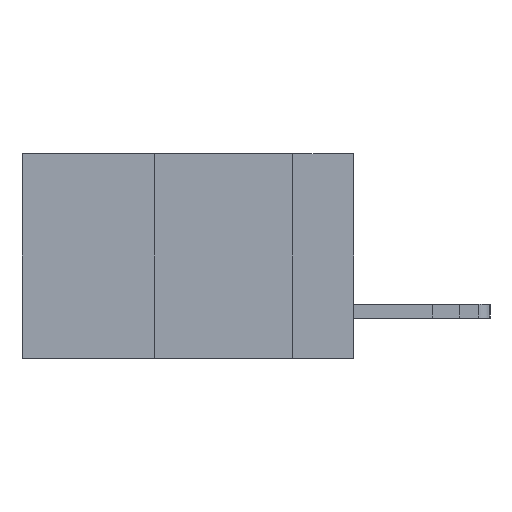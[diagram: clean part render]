
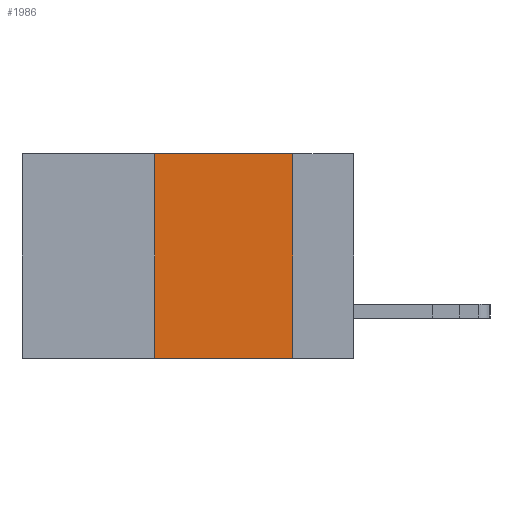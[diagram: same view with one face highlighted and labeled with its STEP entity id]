
A CAD part, left-side view. The second image highlights one B-rep face of the part: STEP entity #1986.
In plain terms, the highlighted planar face has unit normal (-1, 0, 0).
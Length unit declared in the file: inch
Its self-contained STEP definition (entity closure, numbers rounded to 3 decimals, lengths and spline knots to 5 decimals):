
#179 = LINE ( 'NONE', #14898, #10579 ) ;
#461 = ORIENTED_EDGE ( 'NONE', *, *, #7625, .F. ) ;
#1543 = FACE_OUTER_BOUND ( 'NONE', #2567, .T. ) ;
#1986 = ADVANCED_FACE ( 'NONE', ( #1543 ), #6241, .F. ) ;
#2121 = CARTESIAN_POINT ( 'NONE',  ( 0., 0.36, 0. ) ) ;
#2534 = EDGE_CURVE ( 'NONE', #13975, #15255, #6338, .T. ) ;
#2567 = EDGE_LOOP ( 'NONE', ( #5828, #4543, #461, #7724 ) ) ;
#2624 = DIRECTION ( 'NONE',  ( 1., 0., 0. ) ) ;
#3482 = VERTEX_POINT ( 'NONE', #6280 ) ;
#4543 = ORIENTED_EDGE ( 'NONE', *, *, #2534, .F. ) ;
#5828 = ORIENTED_EDGE ( 'NONE', *, *, #9604, .F. ) ;
#6241 = PLANE ( 'NONE',  #15518 ) ;
#6280 = CARTESIAN_POINT ( 'NONE',  ( 0., 0.11, -0.37 ) ) ;
#6338 = LINE ( 'NONE', #11328, #13417 ) ;
#6560 = CARTESIAN_POINT ( 'NONE',  ( 0., 0.6, 0. ) ) ;
#7625 = EDGE_CURVE ( 'NONE', #9426, #13975, #9489, .T. ) ;
#7724 = ORIENTED_EDGE ( 'NONE', *, *, #10273, .T. ) ;
#7765 = VECTOR ( 'NONE', #13208, 39.37008 ) ;
#8237 = CARTESIAN_POINT ( 'NONE',  ( 0., 0.6, -0.37 ) ) ;
#9426 = VERTEX_POINT ( 'NONE', #15965 ) ;
#9489 = LINE ( 'NONE', #13508, #13115 ) ;
#9604 = EDGE_CURVE ( 'NONE', #15255, #3482, #179, .T. ) ;
#10038 = DIRECTION ( 'NONE',  ( 0., 0., -1. ) ) ;
#10273 = EDGE_CURVE ( 'NONE', #9426, #3482, #10732, .T. ) ;
#10579 = VECTOR ( 'NONE', #10038, 39.37008 ) ;
#10732 = LINE ( 'NONE', #8237, #7765 ) ;
#11328 = CARTESIAN_POINT ( 'NONE',  ( 0., 0.6, 0. ) ) ;
#11562 = DIRECTION ( 'NONE',  ( 0., 0., -1. ) ) ;
#11994 = CARTESIAN_POINT ( 'NONE',  ( 0., 0.11, 0. ) ) ;
#13115 = VECTOR ( 'NONE', #14753, 39.37008 ) ;
#13208 = DIRECTION ( 'NONE',  ( 0., -1., 0. ) ) ;
#13417 = VECTOR ( 'NONE', #15108, 39.37008 ) ;
#13508 = CARTESIAN_POINT ( 'NONE',  ( 0., 0.36, 0. ) ) ;
#13975 = VERTEX_POINT ( 'NONE', #2121 ) ;
#14753 = DIRECTION ( 'NONE',  ( 0., 0., 1. ) ) ;
#14898 = CARTESIAN_POINT ( 'NONE',  ( 0., 0.11, 0. ) ) ;
#15108 = DIRECTION ( 'NONE',  ( 0., -1., 0. ) ) ;
#15255 = VERTEX_POINT ( 'NONE', #11994 ) ;
#15518 = AXIS2_PLACEMENT_3D ( 'NONE', #6560, #2624, #11562 ) ;
#15965 = CARTESIAN_POINT ( 'NONE',  ( 0., 0.36, -0.37 ) ) ;
